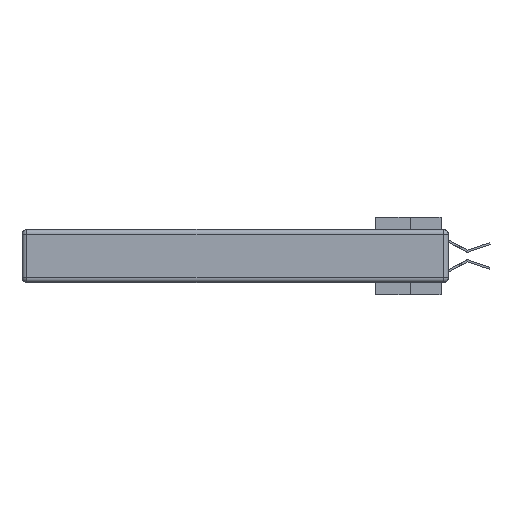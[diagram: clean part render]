
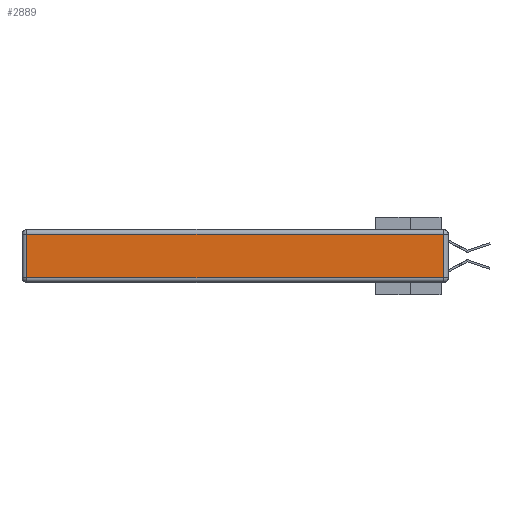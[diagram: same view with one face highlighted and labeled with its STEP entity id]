
A CAD part, left-side view. The second image highlights one B-rep face of the part: STEP entity #2889.
In plain terms, the highlighted planar face has unit normal (-1, 0, 0).
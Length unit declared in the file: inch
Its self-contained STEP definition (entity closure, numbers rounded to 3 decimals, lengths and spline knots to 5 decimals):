
#252 = CARTESIAN_POINT ( 'NONE',  ( 0., 2.72, -0.03 ) ) ;
#362 = ORIENTED_EDGE ( 'NONE', *, *, #21970, .T. ) ;
#1517 = VERTEX_POINT ( 'NONE', #27494 ) ;
#2527 = FACE_OUTER_BOUND ( 'NONE', #2902, .T. ) ;
#2889 = ADVANCED_FACE ( 'NONE', ( #2527 ), #21781, .T. ) ;
#2902 = EDGE_LOOP ( 'NONE', ( #31663, #5934, #362, #17812 ) ) ;
#4853 = CARTESIAN_POINT ( 'NONE',  ( 0., 0., -0.343 ) ) ;
#5932 = DIRECTION ( 'NONE',  ( 0., 0., -1. ) ) ;
#5934 = ORIENTED_EDGE ( 'NONE', *, *, #9640, .T. ) ;
#6983 = LINE ( 'NONE', #16286, #25547 ) ;
#7224 = CARTESIAN_POINT ( 'NONE',  ( 0., 0.03, -0.343 ) ) ;
#8292 = VECTOR ( 'NONE', #5932, 39.37008 ) ;
#8359 = EDGE_CURVE ( 'NONE', #11222, #33542, #33430, .T. ) ;
#8937 = DIRECTION ( 'NONE',  ( 0., -1., 0. ) ) ;
#9640 = EDGE_CURVE ( 'NONE', #1517, #13816, #31719, .T. ) ;
#11222 = VERTEX_POINT ( 'NONE', #252 ) ;
#12203 = DIRECTION ( 'NONE',  ( 0., 0., 1. ) ) ;
#13168 = EDGE_CURVE ( 'NONE', #33542, #1517, #6983, .T. ) ;
#13816 = VERTEX_POINT ( 'NONE', #33590 ) ;
#16286 = CARTESIAN_POINT ( 'NONE',  ( 0., 0., -0.313 ) ) ;
#17047 = CARTESIAN_POINT ( 'NONE',  ( 0., 2.75, -0.03 ) ) ;
#17812 = ORIENTED_EDGE ( 'NONE', *, *, #8359, .T. ) ;
#19751 = VECTOR ( 'NONE', #12203, 39.37008 ) ;
#21781 = PLANE ( 'NONE',  #32166 ) ;
#21970 = EDGE_CURVE ( 'NONE', #13816, #11222, #33343, .T. ) ;
#22147 = CARTESIAN_POINT ( 'NONE',  ( 0., 2.72, -0.343 ) ) ;
#22222 = DIRECTION ( 'NONE',  ( 0., 1., 0. ) ) ;
#22653 = VECTOR ( 'NONE', #22222, 39.37008 ) ;
#25547 = VECTOR ( 'NONE', #8937, 39.37008 ) ;
#26717 = CARTESIAN_POINT ( 'NONE',  ( 0., 2.72, -0.313 ) ) ;
#27494 = CARTESIAN_POINT ( 'NONE',  ( 0., 0.03, -0.313 ) ) ;
#30027 = DIRECTION ( 'NONE',  ( 0., 0., 1. ) ) ;
#31663 = ORIENTED_EDGE ( 'NONE', *, *, #13168, .T. ) ;
#31719 = LINE ( 'NONE', #7224, #19751 ) ;
#32166 = AXIS2_PLACEMENT_3D ( 'NONE', #4853, #32727, #30027 ) ;
#32727 = DIRECTION ( 'NONE',  ( -1., 0., 0. ) ) ;
#33343 = LINE ( 'NONE', #17047, #22653 ) ;
#33430 = LINE ( 'NONE', #22147, #8292 ) ;
#33542 = VERTEX_POINT ( 'NONE', #26717 ) ;
#33590 = CARTESIAN_POINT ( 'NONE',  ( 0., 0.03, -0.03 ) ) ;
